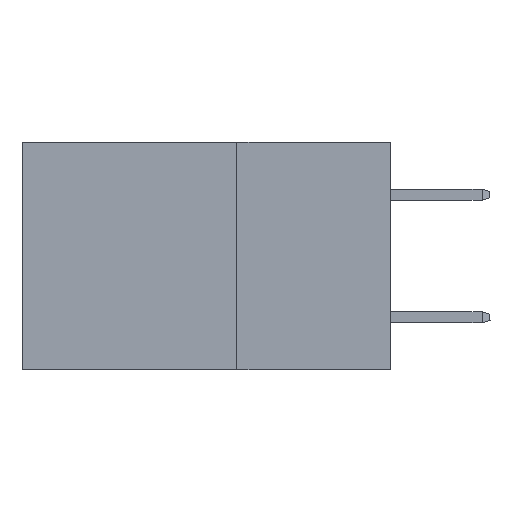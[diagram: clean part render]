
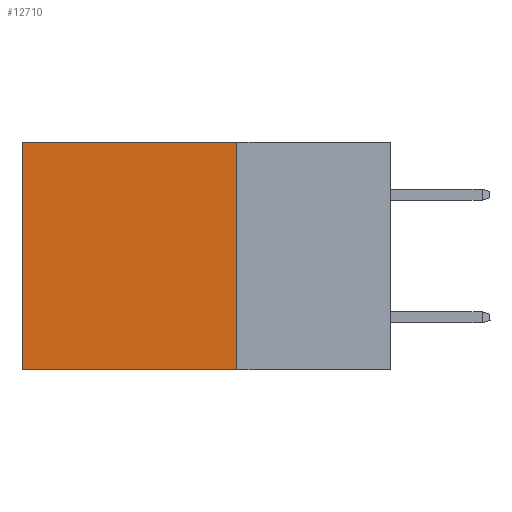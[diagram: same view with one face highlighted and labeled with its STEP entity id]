
A CAD part, left-side view. The second image highlights one B-rep face of the part: STEP entity #12710.
In plain terms, the highlighted planar face has unit normal (-1, 0, 0).
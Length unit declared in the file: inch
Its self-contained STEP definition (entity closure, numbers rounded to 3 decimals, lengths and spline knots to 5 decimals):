
#246 = DIRECTION ( 'NONE',  ( 0., 1., 0. ) ) ;
#622 = EDGE_CURVE ( 'NONE', #14395, #12277, #8006, .T. ) ;
#628 = VECTOR ( 'NONE', #4566, 39.37008 ) ;
#1109 = ORIENTED_EDGE ( 'NONE', *, *, #622, .F. ) ;
#1222 = CARTESIAN_POINT ( 'NONE',  ( 0.2875, 0.25, 0. ) ) ;
#2253 = CARTESIAN_POINT ( 'NONE',  ( 0.2875, 0.6, 0. ) ) ;
#2483 = CARTESIAN_POINT ( 'NONE',  ( 0.2875, 0.25, -0.37 ) ) ;
#2612 = DIRECTION ( 'NONE',  ( 0., 1., 0. ) ) ;
#2669 = FACE_OUTER_BOUND ( 'NONE', #6873, .T. ) ;
#2686 = ORIENTED_EDGE ( 'NONE', *, *, #11379, .T. ) ;
#4009 = CARTESIAN_POINT ( 'NONE',  ( 0.2875, 0.6, 0. ) ) ;
#4066 = VECTOR ( 'NONE', #5441, 39.37008 ) ;
#4566 = DIRECTION ( 'NONE',  ( 0., 0., -1. ) ) ;
#4729 = DIRECTION ( 'NONE',  ( 1., 0., 0. ) ) ;
#4753 = LINE ( 'NONE', #7024, #9045 ) ;
#4755 = VECTOR ( 'NONE', #246, 39.37008 ) ;
#5118 = VERTEX_POINT ( 'NONE', #4009 ) ;
#5441 = DIRECTION ( 'NONE',  ( 0., 0., -1. ) ) ;
#6113 = PLANE ( 'NONE',  #14471 ) ;
#6712 = VERTEX_POINT ( 'NONE', #13090 ) ;
#6873 = EDGE_LOOP ( 'NONE', ( #2686, #7066, #1109, #10319 ) ) ;
#7024 = CARTESIAN_POINT ( 'NONE',  ( 0.2875, 0.25, 0. ) ) ;
#7066 = ORIENTED_EDGE ( 'NONE', *, *, #10374, .F. ) ;
#8006 = LINE ( 'NONE', #1222, #628 ) ;
#9045 = VECTOR ( 'NONE', #2612, 39.37008 ) ;
#9234 = CARTESIAN_POINT ( 'NONE',  ( 0.2875, 0.25, -0.37 ) ) ;
#10319 = ORIENTED_EDGE ( 'NONE', *, *, #13577, .T. ) ;
#10374 = EDGE_CURVE ( 'NONE', #12277, #6712, #12593, .T. ) ;
#11379 = EDGE_CURVE ( 'NONE', #5118, #6712, #14524, .T. ) ;
#12277 = VERTEX_POINT ( 'NONE', #9234 ) ;
#12391 = CARTESIAN_POINT ( 'NONE',  ( 0.2875, 0.25, 0. ) ) ;
#12593 = LINE ( 'NONE', #2483, #4755 ) ;
#12710 = ADVANCED_FACE ( 'NONE', ( #2669 ), #6113, .F. ) ;
#12844 = CARTESIAN_POINT ( 'NONE',  ( 0.2875, 0.25, 0. ) ) ;
#13090 = CARTESIAN_POINT ( 'NONE',  ( 0.2875, 0.6, -0.37 ) ) ;
#13577 = EDGE_CURVE ( 'NONE', #14395, #5118, #4753, .T. ) ;
#13953 = DIRECTION ( 'NONE',  ( 0., 0., -1. ) ) ;
#14395 = VERTEX_POINT ( 'NONE', #12391 ) ;
#14471 = AXIS2_PLACEMENT_3D ( 'NONE', #12844, #4729, #13953 ) ;
#14524 = LINE ( 'NONE', #2253, #4066 ) ;
